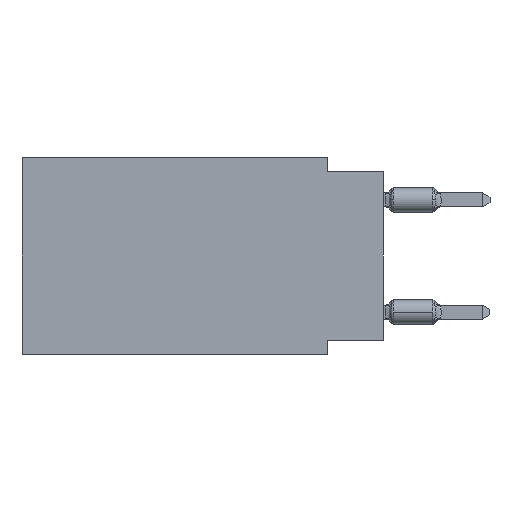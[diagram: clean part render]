
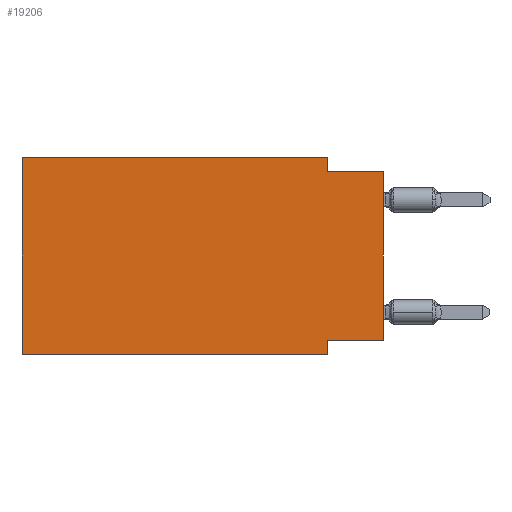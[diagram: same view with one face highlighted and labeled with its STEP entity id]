
A CAD part, left-side view. The second image highlights one B-rep face of the part: STEP entity #19206.
In plain terms, the highlighted planar face has unit normal (-1, 0, 0).
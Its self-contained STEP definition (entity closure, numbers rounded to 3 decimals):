
#458 = LINE ( 'NONE', #20518, #10034 ) ;
#726 = EDGE_CURVE ( 'NONE', #1389, #13141, #11567, .T. ) ;
#767 = CARTESIAN_POINT ( 'NONE',  ( 0., 0., -0.635 ) ) ;
#1389 = VERTEX_POINT ( 'NONE', #11622 ) ;
#1539 = DIRECTION ( 'NONE',  ( 0., -1., 0. ) ) ;
#1642 = VECTOR ( 'NONE', #6576, 1000. ) ;
#2320 = DIRECTION ( 'NONE',  ( 0., -1., 0. ) ) ;
#2909 = CARTESIAN_POINT ( 'NONE',  ( 0., 2.54, -8.255 ) ) ;
#3478 = VECTOR ( 'NONE', #3583, 1000. ) ;
#3581 = ORIENTED_EDGE ( 'NONE', *, *, #6288, .T. ) ;
#3583 = DIRECTION ( 'NONE',  ( 0., -1., 0. ) ) ;
#3681 = VERTEX_POINT ( 'NONE', #767 ) ;
#3920 = DIRECTION ( 'NONE',  ( 0., 0., -1. ) ) ;
#5271 = LINE ( 'NONE', #16901, #1642 ) ;
#5280 = CARTESIAN_POINT ( 'NONE',  ( 0., 16.383, -8.89 ) ) ;
#6288 = EDGE_CURVE ( 'NONE', #15883, #20824, #6847, .T. ) ;
#6326 = CARTESIAN_POINT ( 'NONE',  ( 0., 0., -8.255 ) ) ;
#6449 = EDGE_CURVE ( 'NONE', #18475, #15255, #12517, .T. ) ;
#6576 = DIRECTION ( 'NONE',  ( 0., 0., 1. ) ) ;
#6847 = LINE ( 'NONE', #13379, #3478 ) ;
#7036 = ORIENTED_EDGE ( 'NONE', *, *, #726, .F. ) ;
#7067 = CARTESIAN_POINT ( 'NONE',  ( 0., 0., -8.255 ) ) ;
#7687 = EDGE_CURVE ( 'NONE', #13141, #20487, #8808, .T. ) ;
#8286 = CARTESIAN_POINT ( 'NONE',  ( 0., 16.383, 0. ) ) ;
#8808 = LINE ( 'NONE', #19146, #20052 ) ;
#8968 = ORIENTED_EDGE ( 'NONE', *, *, #7687, .F. ) ;
#9420 = PLANE ( 'NONE',  #21491 ) ;
#9619 = LINE ( 'NONE', #19209, #13898 ) ;
#10034 = VECTOR ( 'NONE', #2320, 1000. ) ;
#10074 = ORIENTED_EDGE ( 'NONE', *, *, #19332, .T. ) ;
#10346 = LINE ( 'NONE', #12194, #13457 ) ;
#10353 = VECTOR ( 'NONE', #1539, 1000. ) ;
#10567 = DIRECTION ( 'NONE',  ( 0., 1., 0. ) ) ;
#11024 = ORIENTED_EDGE ( 'NONE', *, *, #19482, .F. ) ;
#11376 = DIRECTION ( 'NONE',  ( 0., 0., -1. ) ) ;
#11567 = LINE ( 'NONE', #8286, #10353 ) ;
#11622 = CARTESIAN_POINT ( 'NONE',  ( 0., 16.383, 0. ) ) ;
#12194 = CARTESIAN_POINT ( 'NONE',  ( 0., 16.383, 0. ) ) ;
#12517 = LINE ( 'NONE', #7067, #18785 ) ;
#12684 = FACE_OUTER_BOUND ( 'NONE', #20615, .T. ) ;
#12784 = ORIENTED_EDGE ( 'NONE', *, *, #17879, .F. ) ;
#13024 = CARTESIAN_POINT ( 'NONE',  ( 0., 2.54, -0.635 ) ) ;
#13141 = VERTEX_POINT ( 'NONE', #21163 ) ;
#13379 = CARTESIAN_POINT ( 'NONE',  ( 0., 16.383, -8.89 ) ) ;
#13457 = VECTOR ( 'NONE', #13608, 1000. ) ;
#13534 = ORIENTED_EDGE ( 'NONE', *, *, #13807, .F. ) ;
#13608 = DIRECTION ( 'NONE',  ( 0., 0., 1. ) ) ;
#13807 = EDGE_CURVE ( 'NONE', #15883, #1389, #10346, .T. ) ;
#13898 = VECTOR ( 'NONE', #14399, 1000. ) ;
#14399 = DIRECTION ( 'NONE',  ( 0., 0., -1. ) ) ;
#14604 = CARTESIAN_POINT ( 'NONE',  ( 0., 2.54, -8.89 ) ) ;
#14628 = DIRECTION ( 'NONE',  ( 1., 0., 0. ) ) ;
#15205 = ORIENTED_EDGE ( 'NONE', *, *, #6449, .F. ) ;
#15255 = VERTEX_POINT ( 'NONE', #2909 ) ;
#15883 = VERTEX_POINT ( 'NONE', #5280 ) ;
#16901 = CARTESIAN_POINT ( 'NONE',  ( 0., 0., 0. ) ) ;
#17879 = EDGE_CURVE ( 'NONE', #15255, #20824, #9619, .T. ) ;
#18475 = VERTEX_POINT ( 'NONE', #6326 ) ;
#18785 = VECTOR ( 'NONE', #10567, 1000. ) ;
#19146 = CARTESIAN_POINT ( 'NONE',  ( 0., 2.54, 0. ) ) ;
#19206 = ADVANCED_FACE ( 'NONE', ( #12684 ), #9420, .F. ) ;
#19209 = CARTESIAN_POINT ( 'NONE',  ( 0., 2.54, -8.89 ) ) ;
#19211 = CARTESIAN_POINT ( 'NONE',  ( 0., 16.383, 0. ) ) ;
#19332 = EDGE_CURVE ( 'NONE', #18475, #3681, #5271, .T. ) ;
#19482 = EDGE_CURVE ( 'NONE', #20487, #3681, #458, .T. ) ;
#20052 = VECTOR ( 'NONE', #3920, 1000. ) ;
#20487 = VERTEX_POINT ( 'NONE', #13024 ) ;
#20518 = CARTESIAN_POINT ( 'NONE',  ( 0., 0., -0.635 ) ) ;
#20615 = EDGE_LOOP ( 'NONE', ( #10074, #11024, #8968, #7036, #13534, #3581, #12784, #15205 ) ) ;
#20824 = VERTEX_POINT ( 'NONE', #14604 ) ;
#21163 = CARTESIAN_POINT ( 'NONE',  ( 0., 2.54, 0. ) ) ;
#21491 = AXIS2_PLACEMENT_3D ( 'NONE', #19211, #14628, #11376 ) ;
